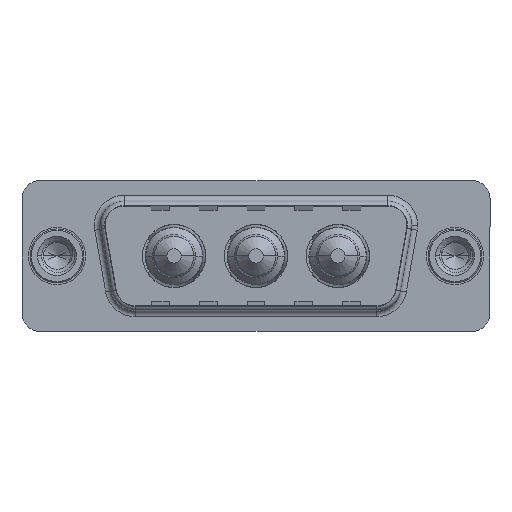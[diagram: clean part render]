
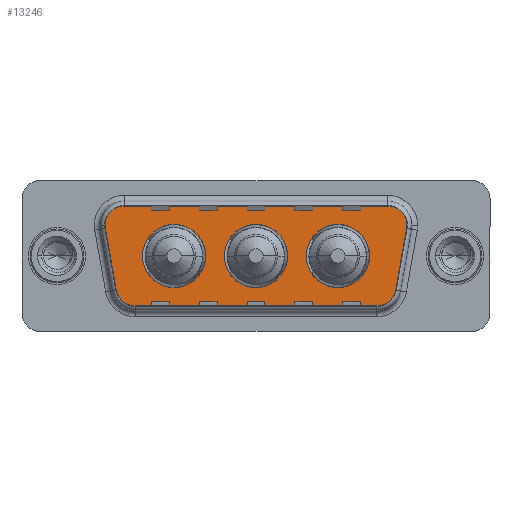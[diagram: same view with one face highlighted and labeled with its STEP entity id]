
A CAD part, top view. The second image highlights one B-rep face of the part: STEP entity #13246.
In plain terms, the highlighted planar face has unit normal (0, 0, 1).
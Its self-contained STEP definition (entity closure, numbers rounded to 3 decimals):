
#66 = ORIENTED_EDGE ( 'NONE', *, *, #6562, .T. ) ;
#108 = EDGE_CURVE ( 'NONE', #8548, #10669, #9383, .T. ) ;
#282 = EDGE_CURVE ( 'NONE', #12857, #1524, #1475, .T. ) ;
#335 = FACE_BOUND ( 'NONE', #9431, .T. ) ;
#466 = VERTEX_POINT ( 'NONE', #4196 ) ;
#496 = CARTESIAN_POINT ( 'NONE',  ( 5.411, 4.9, 0. ) ) ;
#676 = EDGE_CURVE ( 'NONE', #11787, #10440, #6323, .T. ) ;
#841 = DIRECTION ( 'NONE',  ( 1., 0., 0. ) ) ;
#850 = EDGE_CURVE ( 'NONE', #11046, #3686, #4874, .T. ) ;
#1051 = DIRECTION ( 'NONE',  ( 0., 0., 1. ) ) ;
#1223 = CIRCLE ( 'NONE', #14313, 2. ) ;
#1279 = CARTESIAN_POINT ( 'NONE',  ( 6.434, -2.9, 0. ) ) ;
#1360 = ORIENTED_EDGE ( 'NONE', *, *, #13124, .T. ) ;
#1436 = DIRECTION ( 'NONE',  ( 0., 0., 1. ) ) ;
#1475 = CIRCLE ( 'NONE', #13029, 2.65 ) ;
#1524 = VERTEX_POINT ( 'NONE', #5219 ) ;
#1546 = VERTEX_POINT ( 'NONE', #3823 ) ;
#1572 = CIRCLE ( 'NONE', #8178, 2.65 ) ;
#1580 = AXIS2_PLACEMENT_3D ( 'NONE', #3361, #6557, #7724 ) ;
#1716 = EDGE_CURVE ( 'NONE', #466, #13327, #13275, .T. ) ;
#1800 = CIRCLE ( 'NONE', #7934, 2.65 ) ;
#1878 = AXIS2_PLACEMENT_3D ( 'NONE', #1279, #9292, #2409 ) ;
#1970 = CARTESIAN_POINT ( 'NONE',  ( 5.411, 4.9, 0. ) ) ;
#2409 = DIRECTION ( 'NONE',  ( -1., 0., 0. ) ) ;
#2436 = ORIENTED_EDGE ( 'NONE', *, *, #6454, .T. ) ;
#2596 = PLANE ( 'NONE',  #13337 ) ;
#2626 = ORIENTED_EDGE ( 'NONE', *, *, #3690, .F. ) ;
#2679 = DIRECTION ( 'NONE',  ( 1., 0., 0. ) ) ;
#3221 = VECTOR ( 'NONE', #2679, 1000. ) ;
#3325 = VERTEX_POINT ( 'NONE', #1970 ) ;
#3361 = CARTESIAN_POINT ( 'NONE',  ( 16.65, 0., 0. ) ) ;
#3408 = AXIS2_PLACEMENT_3D ( 'NONE', #10599, #12338, #9835 ) ;
#3426 = DIRECTION ( 'NONE',  ( 0.174, 0.985, 0. ) ) ;
#3559 = ORIENTED_EDGE ( 'NONE', *, *, #7395, .F. ) ;
#3605 = DIRECTION ( 'NONE',  ( -1., 0., 0. ) ) ;
#3686 = VERTEX_POINT ( 'NONE', #4941 ) ;
#3690 = EDGE_CURVE ( 'NONE', #13327, #466, #3944, .T. ) ;
#3746 = CARTESIAN_POINT ( 'NONE',  ( 26.866, -2.9, 0. ) ) ;
#3823 = CARTESIAN_POINT ( 'NONE',  ( 27.889, 4.9, 0. ) ) ;
#3944 = CIRCLE ( 'NONE', #3408, 2.65 ) ;
#3977 = DIRECTION ( 'NONE',  ( 0., 0., 1. ) ) ;
#4196 = CARTESIAN_POINT ( 'NONE',  ( 19.3, 0., 0. ) ) ;
#4380 = CIRCLE ( 'NONE', #14529, 2. ) ;
#4409 = EDGE_CURVE ( 'NONE', #1546, #3325, #14612, .T. ) ;
#4589 = CARTESIAN_POINT ( 'NONE',  ( 23.5, 0., 0. ) ) ;
#4726 = AXIS2_PLACEMENT_3D ( 'NONE', #10860, #3977, #11978 ) ;
#4874 = LINE ( 'NONE', #11526, #13585 ) ;
#4941 = CARTESIAN_POINT ( 'NONE',  ( 29.859, 2.553, 0. ) ) ;
#5155 = DIRECTION ( 'NONE',  ( 0.174, -0.985, 0. ) ) ;
#5219 = CARTESIAN_POINT ( 'NONE',  ( 12.45, 0., 0. ) ) ;
#5356 = CARTESIAN_POINT ( 'NONE',  ( 4.464, -3.247, 0. ) ) ;
#5362 = VERTEX_POINT ( 'NONE', #7936 ) ;
#5520 = CARTESIAN_POINT ( 'NONE',  ( 27.889, 2.9, 0. ) ) ;
#5563 = CARTESIAN_POINT ( 'NONE',  ( 3.441, 2.553, 0. ) ) ;
#5772 = DIRECTION ( 'NONE',  ( 1., 0., 0. ) ) ;
#5836 = CARTESIAN_POINT ( 'NONE',  ( 27.889, 2.9, 0. ) ) ;
#5922 = ORIENTED_EDGE ( 'NONE', *, *, #11954, .F. ) ;
#6129 = FACE_BOUND ( 'NONE', #14562, .T. ) ;
#6144 = CARTESIAN_POINT ( 'NONE',  ( 9.8, 0., 0. ) ) ;
#6192 = CARTESIAN_POINT ( 'NONE',  ( 26.866, -4.9, 0. ) ) ;
#6323 = LINE ( 'NONE', #13602, #3221 ) ;
#6338 = VECTOR ( 'NONE', #5155, 1000. ) ;
#6454 = EDGE_CURVE ( 'NONE', #3325, #8548, #11767, .T. ) ;
#6557 = DIRECTION ( 'NONE',  ( 0., 0., 1. ) ) ;
#6562 = EDGE_CURVE ( 'NONE', #3686, #14531, #1223, .T. ) ;
#6583 = ORIENTED_EDGE ( 'NONE', *, *, #9334, .T. ) ;
#6659 = DIRECTION ( 'NONE',  ( -1., 0., 0. ) ) ;
#6671 = ORIENTED_EDGE ( 'NONE', *, *, #850, .T. ) ;
#6972 = DIRECTION ( 'NONE',  ( -1., 0., 0. ) ) ;
#6984 = CARTESIAN_POINT ( 'NONE',  ( 26.15, 0., 0. ) ) ;
#7122 = CIRCLE ( 'NONE', #4726, 2. ) ;
#7395 = EDGE_CURVE ( 'NONE', #1524, #12857, #1572, .T. ) ;
#7723 = DIRECTION ( 'NONE',  ( 0., 0., 1. ) ) ;
#7724 = DIRECTION ( 'NONE',  ( 1., 0., 0. ) ) ;
#7929 = CARTESIAN_POINT ( 'NONE',  ( 5.411, 2.9, 0. ) ) ;
#7934 = AXIS2_PLACEMENT_3D ( 'NONE', #14498, #7723, #841 ) ;
#7936 = CARTESIAN_POINT ( 'NONE',  ( 20.85, 0., 0. ) ) ;
#8178 = AXIS2_PLACEMENT_3D ( 'NONE', #8298, #1436, #9463 ) ;
#8258 = VECTOR ( 'NONE', #3605, 1000. ) ;
#8277 = EDGE_CURVE ( 'NONE', #10440, #11046, #7122, .T. ) ;
#8298 = CARTESIAN_POINT ( 'NONE',  ( 9.8, 0., 0. ) ) ;
#8327 = ORIENTED_EDGE ( 'NONE', *, *, #4409, .T. ) ;
#8330 = DIRECTION ( 'NONE',  ( 0., 0., 1. ) ) ;
#8334 = CARTESIAN_POINT ( 'NONE',  ( 29.889, 2.9, 0. ) ) ;
#8548 = VERTEX_POINT ( 'NONE', #10602 ) ;
#9018 = AXIS2_PLACEMENT_3D ( 'NONE', #7929, #1051, #9071 ) ;
#9071 = DIRECTION ( 'NONE',  ( 1., 0., 0. ) ) ;
#9102 = ORIENTED_EDGE ( 'NONE', *, *, #12724, .F. ) ;
#9292 = DIRECTION ( 'NONE',  ( 0., 0., 1. ) ) ;
#9334 = EDGE_CURVE ( 'NONE', #14531, #1546, #4380, .T. ) ;
#9383 = LINE ( 'NONE', #5563, #6338 ) ;
#9431 = EDGE_LOOP ( 'NONE', ( #3559, #13769 ) ) ;
#9463 = DIRECTION ( 'NONE',  ( 1., 0., 0. ) ) ;
#9672 = EDGE_LOOP ( 'NONE', ( #9674, #6671, #66, #6583, #8327, #2436, #13081, #1360, #10561 ) ) ;
#9674 = ORIENTED_EDGE ( 'NONE', *, *, #8277, .T. ) ;
#9835 = DIRECTION ( 'NONE',  ( 1., 0., 0. ) ) ;
#9925 = EDGE_LOOP ( 'NONE', ( #5922, #9102 ) ) ;
#10440 = VERTEX_POINT ( 'NONE', #6192 ) ;
#10561 = ORIENTED_EDGE ( 'NONE', *, *, #676, .T. ) ;
#10599 = CARTESIAN_POINT ( 'NONE',  ( 16.65, 0., 0. ) ) ;
#10602 = CARTESIAN_POINT ( 'NONE',  ( 3.441, 2.553, 0. ) ) ;
#10669 = VERTEX_POINT ( 'NONE', #5356 ) ;
#10781 = CARTESIAN_POINT ( 'NONE',  ( 14., 0., 0. ) ) ;
#10860 = CARTESIAN_POINT ( 'NONE',  ( 26.866, -2.9, 0. ) ) ;
#11046 = VERTEX_POINT ( 'NONE', #13054 ) ;
#11446 = CIRCLE ( 'NONE', #11650, 2.65 ) ;
#11526 = CARTESIAN_POINT ( 'NONE',  ( 29.859, 2.553, 0. ) ) ;
#11650 = AXIS2_PLACEMENT_3D ( 'NONE', #4589, #12554, #5772 ) ;
#11767 = CIRCLE ( 'NONE', #9018, 2. ) ;
#11787 = VERTEX_POINT ( 'NONE', #14165 ) ;
#11954 = EDGE_CURVE ( 'NONE', #13129, #5362, #1800, .T. ) ;
#11978 = DIRECTION ( 'NONE',  ( 1., 0., 0. ) ) ;
#12129 = FACE_BOUND ( 'NONE', #9925, .T. ) ;
#12338 = DIRECTION ( 'NONE',  ( 0., 0., 1. ) ) ;
#12554 = DIRECTION ( 'NONE',  ( 0., 0., 1. ) ) ;
#12698 = CARTESIAN_POINT ( 'NONE',  ( 7.15, 0., 0. ) ) ;
#12724 = EDGE_CURVE ( 'NONE', #5362, #13129, #11446, .T. ) ;
#12857 = VERTEX_POINT ( 'NONE', #12698 ) ;
#12890 = DIRECTION ( 'NONE',  ( 1., 0., 0. ) ) ;
#13029 = AXIS2_PLACEMENT_3D ( 'NONE', #6144, #14570, #14566 ) ;
#13054 = CARTESIAN_POINT ( 'NONE',  ( 28.836, -3.247, 0. ) ) ;
#13081 = ORIENTED_EDGE ( 'NONE', *, *, #108, .T. ) ;
#13124 = EDGE_CURVE ( 'NONE', #10669, #11787, #13208, .T. ) ;
#13129 = VERTEX_POINT ( 'NONE', #6984 ) ;
#13208 = CIRCLE ( 'NONE', #1878, 2. ) ;
#13246 = ADVANCED_FACE ( 'NONE', ( #6129, #12129, #335, #14762 ), #2596, .T. ) ;
#13275 = CIRCLE ( 'NONE', #1580, 2.65 ) ;
#13327 = VERTEX_POINT ( 'NONE', #10781 ) ;
#13337 = AXIS2_PLACEMENT_3D ( 'NONE', #3746, #8330, #12890 ) ;
#13460 = DIRECTION ( 'NONE',  ( 0., 0., 1. ) ) ;
#13585 = VECTOR ( 'NONE', #3426, 1000. ) ;
#13602 = CARTESIAN_POINT ( 'NONE',  ( 6.434, -4.9, 0. ) ) ;
#13756 = DIRECTION ( 'NONE',  ( 0., 0., 1. ) ) ;
#13769 = ORIENTED_EDGE ( 'NONE', *, *, #282, .F. ) ;
#13831 = ORIENTED_EDGE ( 'NONE', *, *, #1716, .F. ) ;
#14165 = CARTESIAN_POINT ( 'NONE',  ( 6.434, -4.9, 0. ) ) ;
#14313 = AXIS2_PLACEMENT_3D ( 'NONE', #5836, #13756, #6972 ) ;
#14498 = CARTESIAN_POINT ( 'NONE',  ( 23.5, 0., 0. ) ) ;
#14529 = AXIS2_PLACEMENT_3D ( 'NONE', #5520, #13460, #6659 ) ;
#14531 = VERTEX_POINT ( 'NONE', #8334 ) ;
#14562 = EDGE_LOOP ( 'NONE', ( #13831, #2626 ) ) ;
#14566 = DIRECTION ( 'NONE',  ( 1., 0., 0. ) ) ;
#14570 = DIRECTION ( 'NONE',  ( 0., 0., 1. ) ) ;
#14612 = LINE ( 'NONE', #496, #8258 ) ;
#14762 = FACE_OUTER_BOUND ( 'NONE', #9672, .T. ) ;
